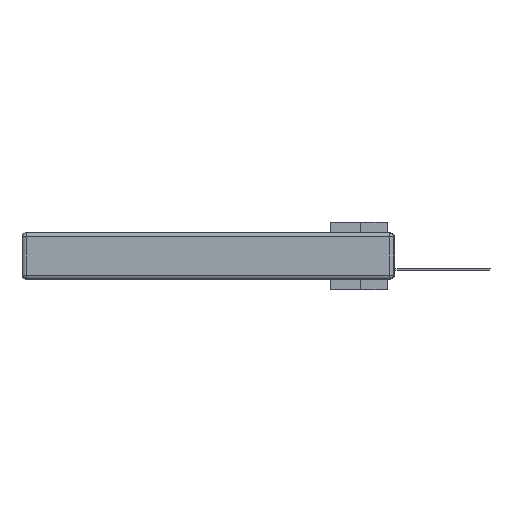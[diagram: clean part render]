
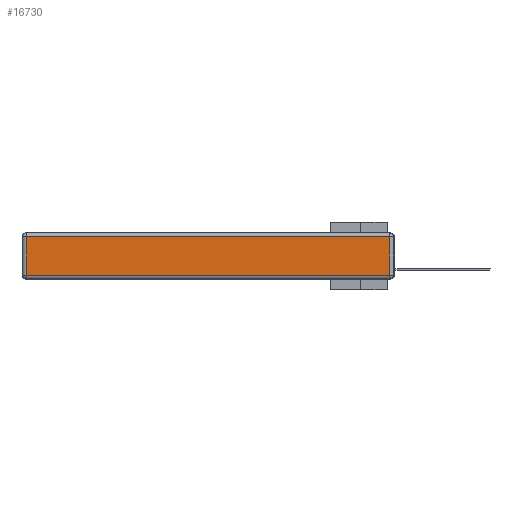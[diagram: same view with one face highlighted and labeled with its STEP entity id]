
A CAD part, left-side view. The second image highlights one B-rep face of the part: STEP entity #16730.
In plain terms, the highlighted planar face has unit normal (-1, 0, 0).
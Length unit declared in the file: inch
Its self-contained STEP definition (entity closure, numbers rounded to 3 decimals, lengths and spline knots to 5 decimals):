
#646 = LINE ( 'NONE', #30088, #22230 ) ;
#2288 = DIRECTION ( 'NONE',  ( 0., 0., -1. ) ) ;
#2565 = CARTESIAN_POINT ( 'NONE',  ( 0., 0.03, -0.03 ) ) ;
#4606 = ORIENTED_EDGE ( 'NONE', *, *, #13088, .T. ) ;
#6428 = ORIENTED_EDGE ( 'NONE', *, *, #31278, .T. ) ;
#6607 = CARTESIAN_POINT ( 'NONE',  ( 0., 0.03, -0.343 ) ) ;
#8883 = FACE_OUTER_BOUND ( 'NONE', #26686, .T. ) ;
#9638 = VERTEX_POINT ( 'NONE', #2565 ) ;
#10762 = CARTESIAN_POINT ( 'NONE',  ( 0., 0., -0.313 ) ) ;
#11681 = VECTOR ( 'NONE', #32456, 39.37008 ) ;
#11737 = CARTESIAN_POINT ( 'NONE',  ( 0., 2.72, -0.03 ) ) ;
#13088 = EDGE_CURVE ( 'NONE', #32747, #26135, #15560, .T. ) ;
#13717 = EDGE_CURVE ( 'NONE', #9638, #32747, #646, .T. ) ;
#15077 = PLANE ( 'NONE',  #34704 ) ;
#15560 = LINE ( 'NONE', #34757, #18239 ) ;
#16286 = VECTOR ( 'NONE', #31611, 39.37008 ) ;
#16392 = DIRECTION ( 'NONE',  ( 0., 1., 0. ) ) ;
#16730 = ADVANCED_FACE ( 'NONE', ( #8883 ), #15077, .T. ) ;
#18239 = VECTOR ( 'NONE', #2288, 39.37008 ) ;
#19706 = DIRECTION ( 'NONE',  ( -1., 0., 0. ) ) ;
#20702 = CARTESIAN_POINT ( 'NONE',  ( 0., 2.72, -0.313 ) ) ;
#22230 = VECTOR ( 'NONE', #16392, 39.37008 ) ;
#22484 = EDGE_CURVE ( 'NONE', #26135, #33059, #29789, .T. ) ;
#23084 = DIRECTION ( 'NONE',  ( 0., 0., 1. ) ) ;
#26135 = VERTEX_POINT ( 'NONE', #20702 ) ;
#26686 = EDGE_LOOP ( 'NONE', ( #26945, #6428, #31077, #4606 ) ) ;
#26945 = ORIENTED_EDGE ( 'NONE', *, *, #22484, .T. ) ;
#28596 = LINE ( 'NONE', #6607, #16286 ) ;
#29789 = LINE ( 'NONE', #10762, #11681 ) ;
#30088 = CARTESIAN_POINT ( 'NONE',  ( 0., 2.75, -0.03 ) ) ;
#30323 = CARTESIAN_POINT ( 'NONE',  ( 0., 0.03, -0.313 ) ) ;
#31077 = ORIENTED_EDGE ( 'NONE', *, *, #13717, .T. ) ;
#31278 = EDGE_CURVE ( 'NONE', #33059, #9638, #28596, .T. ) ;
#31611 = DIRECTION ( 'NONE',  ( 0., 0., 1. ) ) ;
#32456 = DIRECTION ( 'NONE',  ( 0., -1., 0. ) ) ;
#32747 = VERTEX_POINT ( 'NONE', #11737 ) ;
#33059 = VERTEX_POINT ( 'NONE', #30323 ) ;
#33393 = CARTESIAN_POINT ( 'NONE',  ( 0., 0., -0.343 ) ) ;
#34704 = AXIS2_PLACEMENT_3D ( 'NONE', #33393, #19706, #23084 ) ;
#34757 = CARTESIAN_POINT ( 'NONE',  ( 0., 2.72, -0.343 ) ) ;
